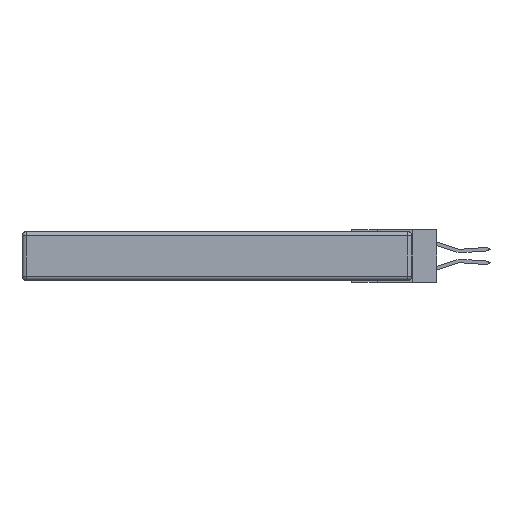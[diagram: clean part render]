
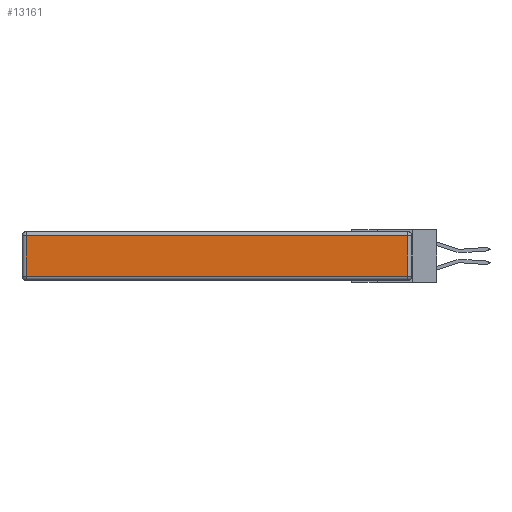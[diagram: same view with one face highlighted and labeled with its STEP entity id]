
A CAD part, left-side view. The second image highlights one B-rep face of the part: STEP entity #13161.
In plain terms, the highlighted planar face has unit normal (-1, 0, 0).
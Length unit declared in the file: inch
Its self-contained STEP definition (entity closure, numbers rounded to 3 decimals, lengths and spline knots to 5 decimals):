
#935 = VERTEX_POINT ( 'NONE', #4490 ) ;
#2715 = CARTESIAN_POINT ( 'NONE',  ( 0., 2.75, -0.03 ) ) ;
#3066 = PLANE ( 'NONE',  #7821 ) ;
#3103 = LINE ( 'NONE', #7214, #12263 ) ;
#3161 = VERTEX_POINT ( 'NONE', #5399 ) ;
#3803 = VECTOR ( 'NONE', #11054, 39.37008 ) ;
#3927 = EDGE_CURVE ( 'NONE', #17145, #3161, #3103, .T. ) ;
#4490 = CARTESIAN_POINT ( 'NONE',  ( 0., 2.72, -0.313 ) ) ;
#4738 = VERTEX_POINT ( 'NONE', #5627 ) ;
#5399 = CARTESIAN_POINT ( 'NONE',  ( 0., 0.03, -0.03 ) ) ;
#5627 = CARTESIAN_POINT ( 'NONE',  ( 0., 2.72, -0.03 ) ) ;
#5848 = CARTESIAN_POINT ( 'NONE',  ( 0., 0., -0.343 ) ) ;
#7136 = CARTESIAN_POINT ( 'NONE',  ( 0., 0.03, -0.313 ) ) ;
#7214 = CARTESIAN_POINT ( 'NONE',  ( 0., 0.03, -0.343 ) ) ;
#7244 = EDGE_CURVE ( 'NONE', #935, #17145, #17098, .T. ) ;
#7821 = AXIS2_PLACEMENT_3D ( 'NONE', #5848, #15640, #17058 ) ;
#7985 = FACE_OUTER_BOUND ( 'NONE', #12890, .T. ) ;
#8880 = ORIENTED_EDGE ( 'NONE', *, *, #9706, .T. ) ;
#9245 = LINE ( 'NONE', #18070, #3803 ) ;
#9706 = EDGE_CURVE ( 'NONE', #3161, #4738, #14347, .T. ) ;
#9918 = ORIENTED_EDGE ( 'NONE', *, *, #3927, .T. ) ;
#10002 = DIRECTION ( 'NONE',  ( 0., 0., 1. ) ) ;
#10611 = VECTOR ( 'NONE', #15318, 39.37008 ) ;
#10701 = VECTOR ( 'NONE', #14688, 39.37008 ) ;
#10880 = ORIENTED_EDGE ( 'NONE', *, *, #13958, .T. ) ;
#11054 = DIRECTION ( 'NONE',  ( 0., 0., -1. ) ) ;
#12263 = VECTOR ( 'NONE', #10002, 39.37008 ) ;
#12890 = EDGE_LOOP ( 'NONE', ( #16715, #9918, #8880, #10880 ) ) ;
#13161 = ADVANCED_FACE ( 'NONE', ( #7985 ), #3066, .T. ) ;
#13958 = EDGE_CURVE ( 'NONE', #4738, #935, #9245, .T. ) ;
#14347 = LINE ( 'NONE', #2715, #10611 ) ;
#14688 = DIRECTION ( 'NONE',  ( 0., -1., 0. ) ) ;
#15318 = DIRECTION ( 'NONE',  ( 0., 1., 0. ) ) ;
#15640 = DIRECTION ( 'NONE',  ( -1., 0., 0. ) ) ;
#16715 = ORIENTED_EDGE ( 'NONE', *, *, #7244, .T. ) ;
#17058 = DIRECTION ( 'NONE',  ( 0., 0., 1. ) ) ;
#17098 = LINE ( 'NONE', #17335, #10701 ) ;
#17145 = VERTEX_POINT ( 'NONE', #7136 ) ;
#17335 = CARTESIAN_POINT ( 'NONE',  ( 0., 0., -0.313 ) ) ;
#18070 = CARTESIAN_POINT ( 'NONE',  ( 0., 2.72, -0.343 ) ) ;
